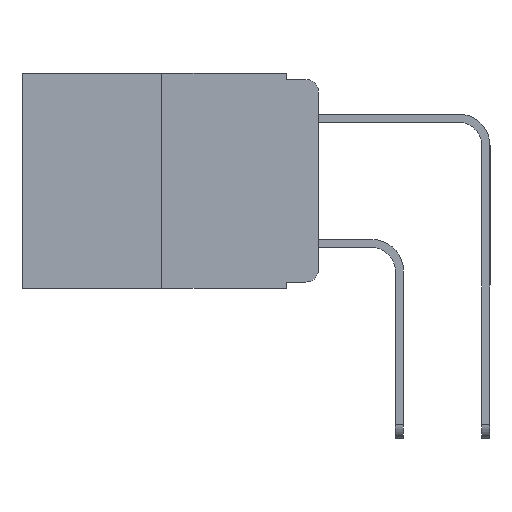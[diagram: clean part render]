
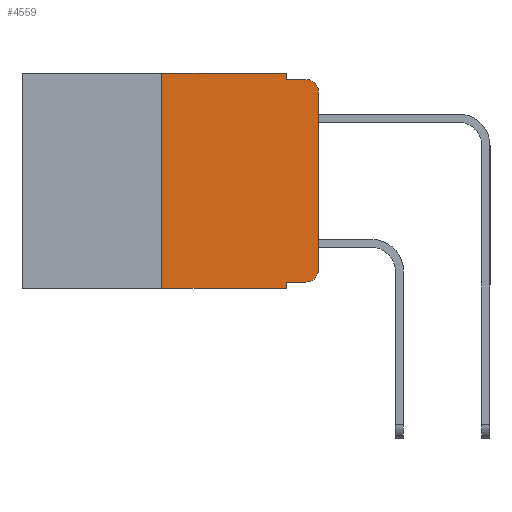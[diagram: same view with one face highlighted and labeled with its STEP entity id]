
A CAD part, left-side view. The second image highlights one B-rep face of the part: STEP entity #4559.
In plain terms, the highlighted planar face has unit normal (-1, 0, 0).
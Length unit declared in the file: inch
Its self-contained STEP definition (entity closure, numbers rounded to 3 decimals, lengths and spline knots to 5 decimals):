
#281 = CARTESIAN_POINT ( 'NONE',  ( 0., 0.25, 0. ) ) ;
#450 = EDGE_CURVE ( 'NONE', #1908, #5381, #9287, .T. ) ;
#647 = VERTEX_POINT ( 'NONE', #12382 ) ;
#1056 = DIRECTION ( 'NONE',  ( 0., 0., -1. ) ) ;
#1097 = CARTESIAN_POINT ( 'NONE',  ( 0., 0.051, 0. ) ) ;
#1672 = CARTESIAN_POINT ( 'NONE',  ( 0., 0.02, -0.333 ) ) ;
#1908 = VERTEX_POINT ( 'NONE', #12314 ) ;
#2024 = VECTOR ( 'NONE', #9730, 39.37008 ) ;
#2057 = CARTESIAN_POINT ( 'NONE',  ( 0., 0.02, -0.03 ) ) ;
#2142 = EDGE_CURVE ( 'NONE', #647, #9384, #16364, .T. ) ;
#2458 = EDGE_CURVE ( 'NONE', #1908, #10737, #4761, .T. ) ;
#2610 = ORIENTED_EDGE ( 'NONE', *, *, #7652, .T. ) ;
#2631 = ORIENTED_EDGE ( 'NONE', *, *, #6720, .T. ) ;
#2636 = ORIENTED_EDGE ( 'NONE', *, *, #2142, .F. ) ;
#2741 = ORIENTED_EDGE ( 'NONE', *, *, #16320, .F. ) ;
#2901 = AXIS2_PLACEMENT_3D ( 'NONE', #16620, #9256, #1056 ) ;
#2968 = DIRECTION ( 'NONE',  ( 0., 0., 1. ) ) ;
#2992 = ORIENTED_EDGE ( 'NONE', *, *, #12124, .F. ) ;
#3121 = LINE ( 'NONE', #8843, #13255 ) ;
#3237 = CARTESIAN_POINT ( 'NONE',  ( 0., 0.02, -0.01 ) ) ;
#3264 = CARTESIAN_POINT ( 'NONE',  ( 0., 0.051, -0.333 ) ) ;
#3273 = EDGE_CURVE ( 'NONE', #16299, #10737, #13179, .T. ) ;
#3322 = ORIENTED_EDGE ( 'NONE', *, *, #3388, .F. ) ;
#3382 = CARTESIAN_POINT ( 'NONE',  ( 0., 0.25, 0. ) ) ;
#3388 = EDGE_CURVE ( 'NONE', #16299, #16571, #4521, .T. ) ;
#3417 = DIRECTION ( 'NONE',  ( 0., 0., -1. ) ) ;
#3489 = CARTESIAN_POINT ( 'NONE',  ( 0., 0.473, -0.343 ) ) ;
#3601 = ORIENTED_EDGE ( 'NONE', *, *, #3273, .T. ) ;
#3746 = ORIENTED_EDGE ( 'NONE', *, *, #2458, .F. ) ;
#3838 = ORIENTED_EDGE ( 'NONE', *, *, #450, .T. ) ;
#4028 = CARTESIAN_POINT ( 'NONE',  ( 0., 0., -0.313 ) ) ;
#4063 = DIRECTION ( 'NONE',  ( 0., -1., 0. ) ) ;
#4078 = ORIENTED_EDGE ( 'NONE', *, *, #15703, .T. ) ;
#4521 = LINE ( 'NONE', #3382, #8159 ) ;
#4559 = ADVANCED_FACE ( 'NONE', ( #5150 ), #13239, .F. ) ;
#4761 = LINE ( 'NONE', #14747, #5198 ) ;
#5150 = FACE_OUTER_BOUND ( 'NONE', #12728, .T. ) ;
#5198 = VECTOR ( 'NONE', #9306, 39.37008 ) ;
#5208 = CARTESIAN_POINT ( 'NONE',  ( 0., 0.25, -0.343 ) ) ;
#5381 = VERTEX_POINT ( 'NONE', #1672 ) ;
#5426 = CARTESIAN_POINT ( 'NONE',  ( 0., 0.473, 0. ) ) ;
#5685 = LINE ( 'NONE', #14644, #2024 ) ;
#6151 = VECTOR ( 'NONE', #8975, 39.37008 ) ;
#6720 = EDGE_CURVE ( 'NONE', #16132, #9384, #16829, .T. ) ;
#6785 = DIRECTION ( 'NONE',  ( 1., 0., 0. ) ) ;
#6908 = LINE ( 'NONE', #1097, #10047 ) ;
#7652 = EDGE_CURVE ( 'NONE', #15386, #16132, #3121, .T. ) ;
#7723 = AXIS2_PLACEMENT_3D ( 'NONE', #5426, #6785, #15621 ) ;
#8159 = VECTOR ( 'NONE', #2968, 39.37008 ) ;
#8843 = CARTESIAN_POINT ( 'NONE',  ( 0., 0., 0. ) ) ;
#8975 = DIRECTION ( 'NONE',  ( 0., -1., 0. ) ) ;
#9256 = DIRECTION ( 'NONE',  ( -1., 0., 0. ) ) ;
#9287 = LINE ( 'NONE', #3264, #6151 ) ;
#9306 = DIRECTION ( 'NONE',  ( 0., 0., -1. ) ) ;
#9384 = VERTEX_POINT ( 'NONE', #3237 ) ;
#9685 = CARTESIAN_POINT ( 'NONE',  ( 0., 0.051, -0.01 ) ) ;
#9730 = DIRECTION ( 'NONE',  ( 0., -1., 0. ) ) ;
#9847 = VECTOR ( 'NONE', #4063, 39.37008 ) ;
#9857 = VECTOR ( 'NONE', #15022, 39.37008 ) ;
#10047 = VECTOR ( 'NONE', #13059, 39.37008 ) ;
#10737 = VERTEX_POINT ( 'NONE', #13017 ) ;
#11428 = CARTESIAN_POINT ( 'NONE',  ( 0., 0., -0.03 ) ) ;
#11435 = DIRECTION ( 'NONE',  ( -1., 0., 0. ) ) ;
#11833 = VERTEX_POINT ( 'NONE', #15339 ) ;
#12124 = EDGE_CURVE ( 'NONE', #16571, #11833, #5685, .T. ) ;
#12314 = CARTESIAN_POINT ( 'NONE',  ( 0., 0.051, -0.333 ) ) ;
#12382 = CARTESIAN_POINT ( 'NONE',  ( 0., 0.051, -0.01 ) ) ;
#12728 = EDGE_LOOP ( 'NONE', ( #2610, #2631, #2636, #2741, #2992, #3322, #3601, #3746, #3838, #4078 ) ) ;
#13017 = CARTESIAN_POINT ( 'NONE',  ( 0., 0.051, -0.343 ) ) ;
#13059 = DIRECTION ( 'NONE',  ( 0., 0., -1. ) ) ;
#13179 = LINE ( 'NONE', #3489, #9847 ) ;
#13204 = CIRCLE ( 'NONE', #2901, 0.02 ) ;
#13239 = PLANE ( 'NONE',  #7723 ) ;
#13255 = VECTOR ( 'NONE', #15061, 39.37008 ) ;
#14644 = CARTESIAN_POINT ( 'NONE',  ( 0., 0.473, 0. ) ) ;
#14747 = CARTESIAN_POINT ( 'NONE',  ( 0., 0.051, 0. ) ) ;
#15022 = DIRECTION ( 'NONE',  ( 0., -1., 0. ) ) ;
#15030 = AXIS2_PLACEMENT_3D ( 'NONE', #2057, #11435, #3417 ) ;
#15061 = DIRECTION ( 'NONE',  ( 0., 0., 1. ) ) ;
#15339 = CARTESIAN_POINT ( 'NONE',  ( 0., 0.051, 0. ) ) ;
#15386 = VERTEX_POINT ( 'NONE', #4028 ) ;
#15621 = DIRECTION ( 'NONE',  ( 0., 0., -1. ) ) ;
#15703 = EDGE_CURVE ( 'NONE', #5381, #15386, #13204, .T. ) ;
#16132 = VERTEX_POINT ( 'NONE', #11428 ) ;
#16299 = VERTEX_POINT ( 'NONE', #5208 ) ;
#16320 = EDGE_CURVE ( 'NONE', #11833, #647, #6908, .T. ) ;
#16364 = LINE ( 'NONE', #9685, #9857 ) ;
#16571 = VERTEX_POINT ( 'NONE', #281 ) ;
#16620 = CARTESIAN_POINT ( 'NONE',  ( 0., 0.02, -0.313 ) ) ;
#16829 = CIRCLE ( 'NONE', #15030, 0.02 ) ;
